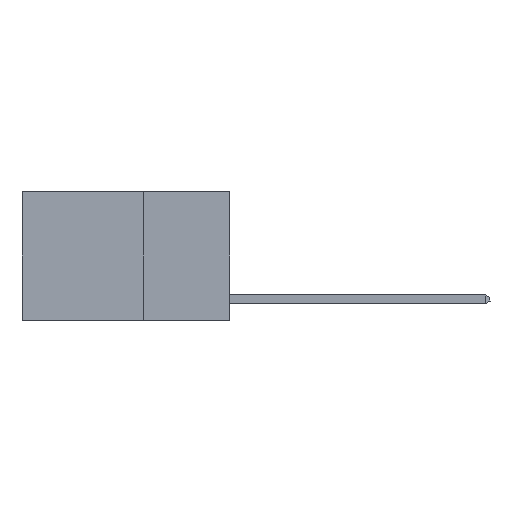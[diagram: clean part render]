
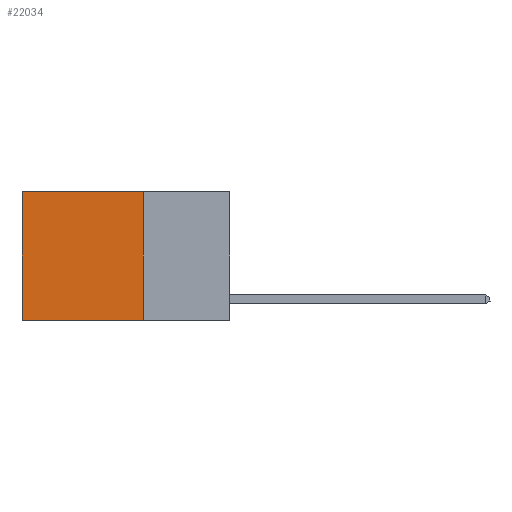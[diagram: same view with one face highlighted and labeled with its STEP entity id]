
A CAD part, left-side view. The second image highlights one B-rep face of the part: STEP entity #22034.
In plain terms, the highlighted planar face has unit normal (-1, 0, 0).
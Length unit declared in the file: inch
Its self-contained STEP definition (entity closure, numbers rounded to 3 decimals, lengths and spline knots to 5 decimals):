
#1246 = EDGE_CURVE ( 'NONE', #18702, #22967, #20375, .T. ) ;
#1894 = CARTESIAN_POINT ( 'NONE',  ( 0.2625, 0.25, 0. ) ) ;
#2124 = CARTESIAN_POINT ( 'NONE',  ( 0.2625, 0.6, -0.37 ) ) ;
#2702 = LINE ( 'NONE', #3070, #23027 ) ;
#3070 = CARTESIAN_POINT ( 'NONE',  ( 0.2625, 0.25, -0.37 ) ) ;
#3240 = CARTESIAN_POINT ( 'NONE',  ( 0.2625, 0.6, 0. ) ) ;
#4564 = ORIENTED_EDGE ( 'NONE', *, *, #22475, .F. ) ;
#4862 = DIRECTION ( 'NONE',  ( 0., 1., 0. ) ) ;
#5645 = EDGE_LOOP ( 'NONE', ( #7437, #4564, #14144, #22635 ) ) ;
#5856 = VECTOR ( 'NONE', #9486, 39.37008 ) ;
#7227 = CARTESIAN_POINT ( 'NONE',  ( 0.2625, 0.25, 0. ) ) ;
#7437 = ORIENTED_EDGE ( 'NONE', *, *, #1246, .T. ) ;
#7892 = DIRECTION ( 'NONE',  ( 0., 1., 0. ) ) ;
#9486 = DIRECTION ( 'NONE',  ( 0., 0., -1. ) ) ;
#9857 = VERTEX_POINT ( 'NONE', #22052 ) ;
#10667 = FACE_OUTER_BOUND ( 'NONE', #5645, .T. ) ;
#12297 = CARTESIAN_POINT ( 'NONE',  ( 0.2625, 0.25, 0. ) ) ;
#13176 = CARTESIAN_POINT ( 'NONE',  ( 0.2625, 0.6, 0. ) ) ;
#14144 = ORIENTED_EDGE ( 'NONE', *, *, #22251, .F. ) ;
#16090 = PLANE ( 'NONE',  #22303 ) ;
#18233 = VERTEX_POINT ( 'NONE', #20175 ) ;
#18702 = VERTEX_POINT ( 'NONE', #13176 ) ;
#18876 = EDGE_CURVE ( 'NONE', #9857, #18702, #23584, .T. ) ;
#20175 = CARTESIAN_POINT ( 'NONE',  ( 0.2625, 0.25, -0.37 ) ) ;
#20375 = LINE ( 'NONE', #3240, #5856 ) ;
#21851 = VECTOR ( 'NONE', #7892, 39.37008 ) ;
#22034 = ADVANCED_FACE ( 'NONE', ( #10667 ), #16090, .F. ) ;
#22052 = CARTESIAN_POINT ( 'NONE',  ( 0.2625, 0.25, 0. ) ) ;
#22251 = EDGE_CURVE ( 'NONE', #9857, #18233, #23641, .T. ) ;
#22303 = AXIS2_PLACEMENT_3D ( 'NONE', #12297, #23734, #23577 ) ;
#22471 = VECTOR ( 'NONE', #22661, 39.37008 ) ;
#22475 = EDGE_CURVE ( 'NONE', #18233, #22967, #2702, .T. ) ;
#22635 = ORIENTED_EDGE ( 'NONE', *, *, #18876, .T. ) ;
#22661 = DIRECTION ( 'NONE',  ( 0., 0., -1. ) ) ;
#22967 = VERTEX_POINT ( 'NONE', #2124 ) ;
#23027 = VECTOR ( 'NONE', #4862, 39.37008 ) ;
#23577 = DIRECTION ( 'NONE',  ( 0., 0., -1. ) ) ;
#23584 = LINE ( 'NONE', #7227, #21851 ) ;
#23641 = LINE ( 'NONE', #1894, #22471 ) ;
#23734 = DIRECTION ( 'NONE',  ( 1., 0., 0. ) ) ;
